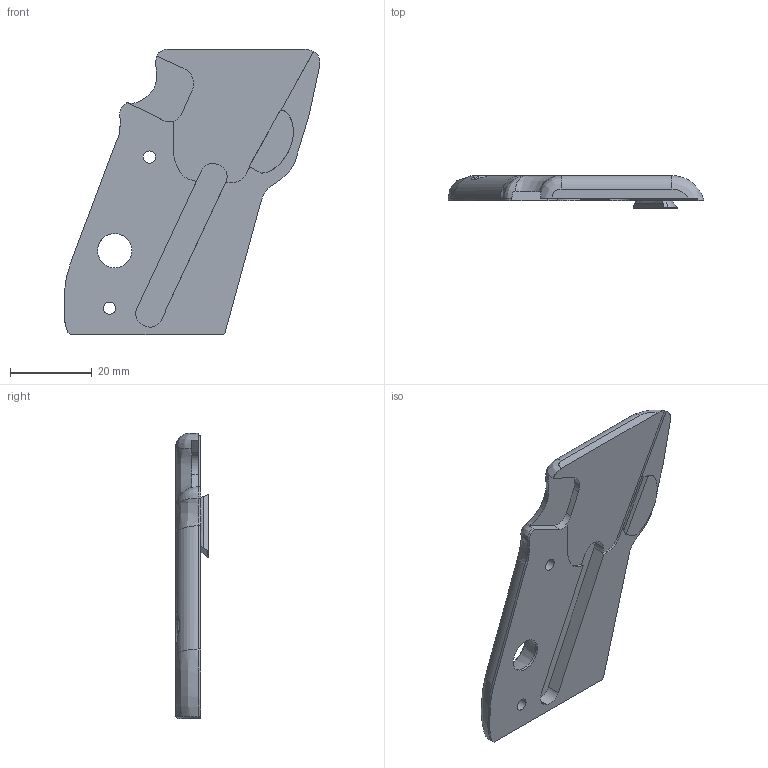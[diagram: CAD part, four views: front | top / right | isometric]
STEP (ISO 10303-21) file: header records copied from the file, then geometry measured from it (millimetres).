
FILE_DESCRIPTION(/* description */ (''),/* implementation_level */ '2;1');
FILE_NAME(/* name */ '21a-Grip-L-Final.step',/* time_stamp */ '2021-11-09T19:44:19-08:00',/* author */ (''),/* organization */ (''),/* preprocessor_version */ 'ST-DEVELOPER v18.1',/* originating_system */ 'Autodesk Translation Framework v10.10.0.1391',/* authorisation */ '');
FILE_SCHEMA (('AUTOMOTIVE_DESIGN { 1 0 10303 214 3 1 1 }'));
Length unit declared in the file: millimetre
Products named in the file (1): Grip-L-Final
Bounding box: 62.7 x 8 x 69.91 mm (x, y, z)
Volume: 13795 mm3; surface area: 7861.4 mm2
Topology: 1 solids, 1 shells, 746 faces, 2053 edges, 1335 vertices
Faces by surface type: plane 367, bspline 331, cylinder 36, torus 7, cone 5
Full cylindrical faces by diameter (mm): 3 x2, 6.2 x2, 7.2 x1, 8.4 x1, 18.002 x1
Entity records: 37326 total; most frequent: CARTESIAN_POINT 20622, ORIENTED_EDGE 4104, DIRECTION 2320, EDGE_CURVE 2052, VERTEX_POINT 1335, LINE 1240, VECTOR 1240, EDGE_LOOP 779
